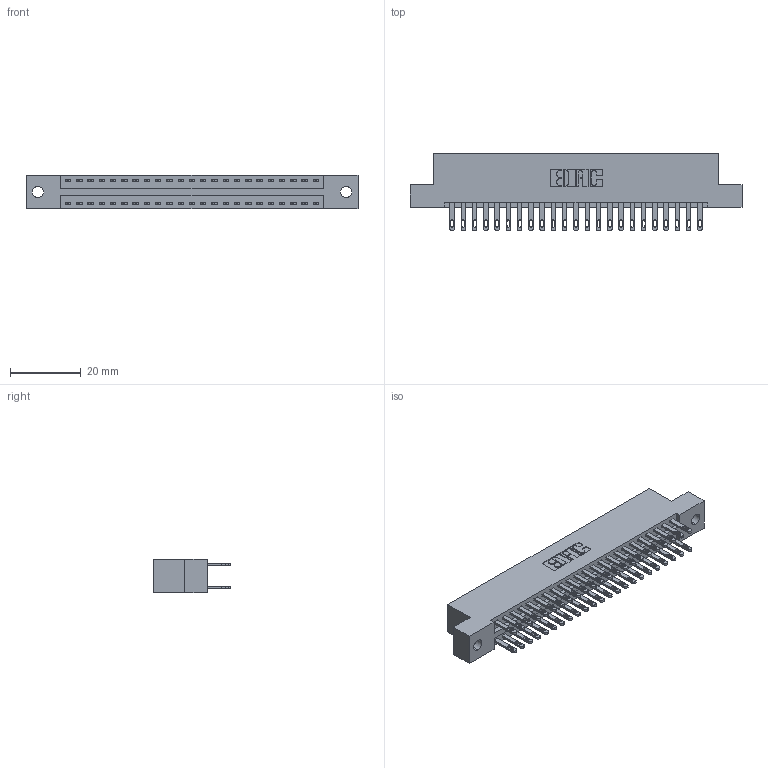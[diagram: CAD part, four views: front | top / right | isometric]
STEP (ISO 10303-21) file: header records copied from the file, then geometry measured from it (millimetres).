
FILE_DESCRIPTION (( 'STEP AP203' ), '1' );
FILE_NAME ('346-046-500-202.STEP', '2022-05-20T08:45:29', ( '' ), ( '' ), 'SwSTEP 2.0', 'SolidWorks 2020', '' );
FILE_SCHEMA (( 'CONFIG_CONTROL_DESIGN' ));
Length unit declared in the file: inch
Products named in the file (3): 345-292-001_345-293-100; 346-046-500-202; 346 Part_Flush Mounting Lugs - 0.128 Dia
Assembly tree (47 placements, depth 2):
  346-046-500-202
    346 Part_Flush Mounting Lugs - 0.128 Dia
    345-292-001_345-293-100  x46
Bounding box: 93.6 x 21.84 x 9.4 mm (x, y, z)
Volume: 9083.4 mm3; surface area: 12399.3 mm2
Topology: 47 solids, 47 shells, 2330 faces, 7091 edges, 4726 vertices
Faces by surface type: plane 1410, cylinder 920
Entity records: 17501 total; most frequent: CARTESIAN_POINT 2908, ORIENTED_EDGE 2842, DIRECTION 2617, EDGE_CURVE 1421, VECTOR 1193, LINE 1193, VERTEX_POINT 946, AXIS2_PLACEMENT_3D 712
